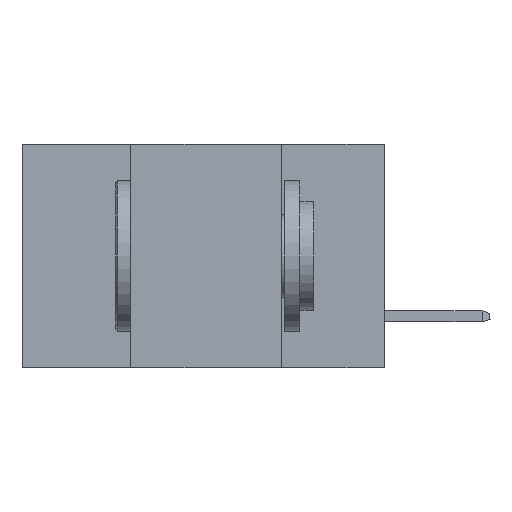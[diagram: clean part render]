
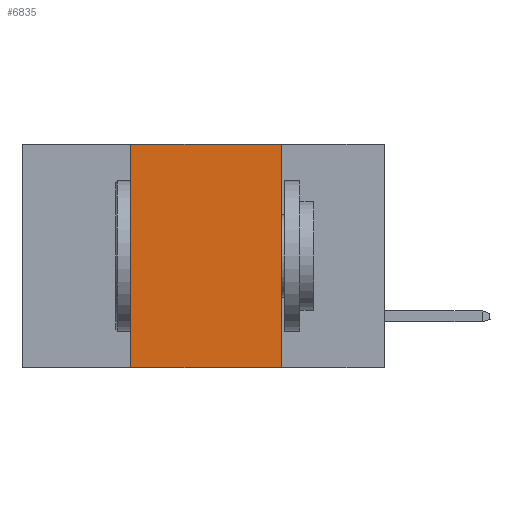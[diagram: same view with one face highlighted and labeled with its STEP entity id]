
A CAD part, left-side view. The second image highlights one B-rep face of the part: STEP entity #6835.
In plain terms, the highlighted planar face has unit normal (-1, 0, 0).
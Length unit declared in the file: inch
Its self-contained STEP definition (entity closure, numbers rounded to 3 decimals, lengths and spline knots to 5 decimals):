
#375 = CARTESIAN_POINT ( 'NONE',  ( 0., 0.17, 0. ) ) ;
#1108 = LINE ( 'NONE', #10326, #8738 ) ;
#1815 = VECTOR ( 'NONE', #8627, 39.37008 ) ;
#1819 = EDGE_CURVE ( 'NONE', #12725, #9262, #3514, .T. ) ;
#2581 = DIRECTION ( 'NONE',  ( 1., 0., 0. ) ) ;
#2956 = DIRECTION ( 'NONE',  ( 0., -1., 0. ) ) ;
#3175 = ORIENTED_EDGE ( 'NONE', *, *, #3425, .F. ) ;
#3425 = EDGE_CURVE ( 'NONE', #4225, #12725, #1108, .T. ) ;
#3455 = DIRECTION ( 'NONE',  ( 0., 0., -1. ) ) ;
#3514 = LINE ( 'NONE', #375, #11603 ) ;
#4149 = ORIENTED_EDGE ( 'NONE', *, *, #7388, .F. ) ;
#4225 = VERTEX_POINT ( 'NONE', #13250 ) ;
#4294 = CARTESIAN_POINT ( 'NONE',  ( 0., 0.42, 0. ) ) ;
#5022 = DIRECTION ( 'NONE',  ( 0., -1., 0. ) ) ;
#5281 = FACE_OUTER_BOUND ( 'NONE', #9941, .T. ) ;
#5580 = AXIS2_PLACEMENT_3D ( 'NONE', #6951, #2581, #12177 ) ;
#6835 = ADVANCED_FACE ( 'NONE', ( #5281 ), #11093, .F. ) ;
#6951 = CARTESIAN_POINT ( 'NONE',  ( 0., 0.6, 0. ) ) ;
#7388 = EDGE_CURVE ( 'NONE', #12742, #4225, #10275, .T. ) ;
#8627 = DIRECTION ( 'NONE',  ( 0., 0., 1. ) ) ;
#8636 = EDGE_CURVE ( 'NONE', #12742, #9262, #13640, .T. ) ;
#8644 = CARTESIAN_POINT ( 'NONE',  ( 0., 0.42, -0.37 ) ) ;
#8738 = VECTOR ( 'NONE', #2956, 39.37008 ) ;
#8747 = CARTESIAN_POINT ( 'NONE',  ( 0., 0.6, -0.37 ) ) ;
#9085 = ORIENTED_EDGE ( 'NONE', *, *, #1819, .F. ) ;
#9262 = VERTEX_POINT ( 'NONE', #13262 ) ;
#9624 = ORIENTED_EDGE ( 'NONE', *, *, #8636, .T. ) ;
#9941 = EDGE_LOOP ( 'NONE', ( #9085, #3175, #4149, #9624 ) ) ;
#10275 = LINE ( 'NONE', #4294, #1815 ) ;
#10326 = CARTESIAN_POINT ( 'NONE',  ( 0., 0.6, 0. ) ) ;
#10493 = CARTESIAN_POINT ( 'NONE',  ( 0., 0.17, 0. ) ) ;
#11093 = PLANE ( 'NONE',  #5580 ) ;
#11603 = VECTOR ( 'NONE', #3455, 39.37008 ) ;
#12177 = DIRECTION ( 'NONE',  ( 0., 0., -1. ) ) ;
#12663 = VECTOR ( 'NONE', #5022, 39.37008 ) ;
#12725 = VERTEX_POINT ( 'NONE', #10493 ) ;
#12742 = VERTEX_POINT ( 'NONE', #8644 ) ;
#13250 = CARTESIAN_POINT ( 'NONE',  ( 0., 0.42, 0. ) ) ;
#13262 = CARTESIAN_POINT ( 'NONE',  ( 0., 0.17, -0.37 ) ) ;
#13640 = LINE ( 'NONE', #8747, #12663 ) ;
